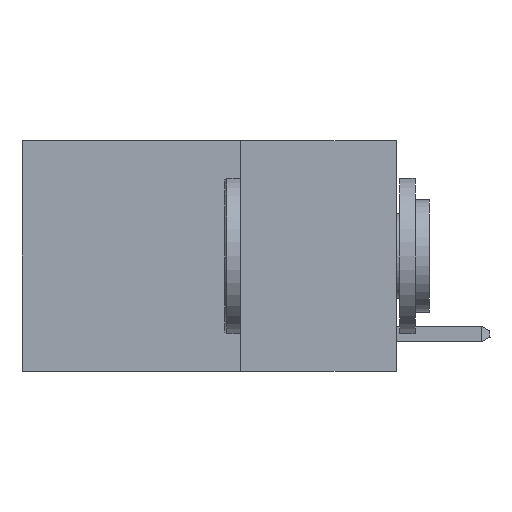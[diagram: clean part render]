
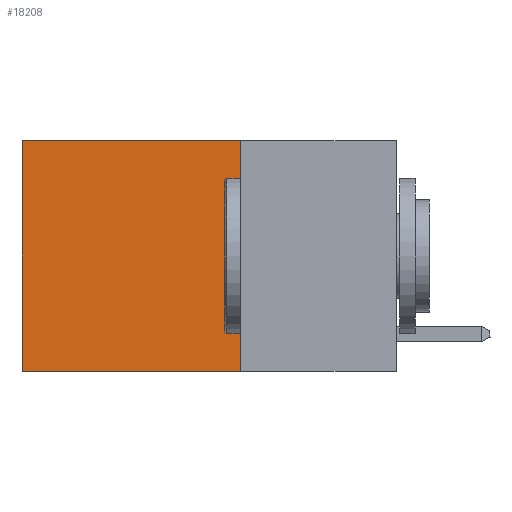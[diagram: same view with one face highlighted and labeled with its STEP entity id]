
A CAD part, left-side view. The second image highlights one B-rep face of the part: STEP entity #18208.
In plain terms, the highlighted planar face has unit normal (-1, 0, 0).
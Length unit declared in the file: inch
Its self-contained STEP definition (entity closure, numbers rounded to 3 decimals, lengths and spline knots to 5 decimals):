
#209 = VERTEX_POINT ( 'NONE', #7022 ) ;
#891 = LINE ( 'NONE', #6782, #5413 ) ;
#1148 = DIRECTION ( 'NONE',  ( 0., 1., 0. ) ) ;
#2080 = CARTESIAN_POINT ( 'NONE',  ( 0.2625, 0.6, -0.37 ) ) ;
#2104 = CARTESIAN_POINT ( 'NONE',  ( 0.2625, 0.25, 0. ) ) ;
#2288 = DIRECTION ( 'NONE',  ( 0., 0., -1. ) ) ;
#2586 = FACE_OUTER_BOUND ( 'NONE', #5736, .T. ) ;
#3307 = EDGE_CURVE ( 'NONE', #209, #12786, #891, .T. ) ;
#4121 = DIRECTION ( 'NONE',  ( 0., 0., -1. ) ) ;
#4512 = EDGE_CURVE ( 'NONE', #18845, #19349, #22147, .T. ) ;
#4823 = ORIENTED_EDGE ( 'NONE', *, *, #24743, .T. ) ;
#5413 = VECTOR ( 'NONE', #1148, 39.37008 ) ;
#5469 = VECTOR ( 'NONE', #8671, 39.37008 ) ;
#5736 = EDGE_LOOP ( 'NONE', ( #4823, #24386, #6861, #17912 ) ) ;
#6782 = CARTESIAN_POINT ( 'NONE',  ( 0.2625, 0.25, -0.37 ) ) ;
#6861 = ORIENTED_EDGE ( 'NONE', *, *, #14968, .F. ) ;
#7022 = CARTESIAN_POINT ( 'NONE',  ( 0.2625, 0.25, -0.37 ) ) ;
#7520 = LINE ( 'NONE', #13370, #19555 ) ;
#8671 = DIRECTION ( 'NONE',  ( 0., 1., 0. ) ) ;
#9626 = AXIS2_PLACEMENT_3D ( 'NONE', #23174, #23422, #4121 ) ;
#12786 = VERTEX_POINT ( 'NONE', #2080 ) ;
#13370 = CARTESIAN_POINT ( 'NONE',  ( 0.2625, 0.25, 0. ) ) ;
#14968 = EDGE_CURVE ( 'NONE', #18845, #209, #7520, .T. ) ;
#15144 = DIRECTION ( 'NONE',  ( 0., 0., -1. ) ) ;
#17912 = ORIENTED_EDGE ( 'NONE', *, *, #4512, .T. ) ;
#18208 = ADVANCED_FACE ( 'NONE', ( #2586 ), #19637, .F. ) ;
#18845 = VERTEX_POINT ( 'NONE', #2104 ) ;
#19349 = VERTEX_POINT ( 'NONE', #21531 ) ;
#19448 = CARTESIAN_POINT ( 'NONE',  ( 0.2625, 0.6, 0. ) ) ;
#19555 = VECTOR ( 'NONE', #15144, 39.37008 ) ;
#19637 = PLANE ( 'NONE',  #9626 ) ;
#20260 = CARTESIAN_POINT ( 'NONE',  ( 0.2625, 0.25, 0. ) ) ;
#21531 = CARTESIAN_POINT ( 'NONE',  ( 0.2625, 0.6, 0. ) ) ;
#22147 = LINE ( 'NONE', #20260, #5469 ) ;
#23174 = CARTESIAN_POINT ( 'NONE',  ( 0.2625, 0.25, 0. ) ) ;
#23235 = LINE ( 'NONE', #19448, #23476 ) ;
#23422 = DIRECTION ( 'NONE',  ( 1., 0., 0. ) ) ;
#23476 = VECTOR ( 'NONE', #2288, 39.37008 ) ;
#24386 = ORIENTED_EDGE ( 'NONE', *, *, #3307, .F. ) ;
#24743 = EDGE_CURVE ( 'NONE', #19349, #12786, #23235, .T. ) ;
